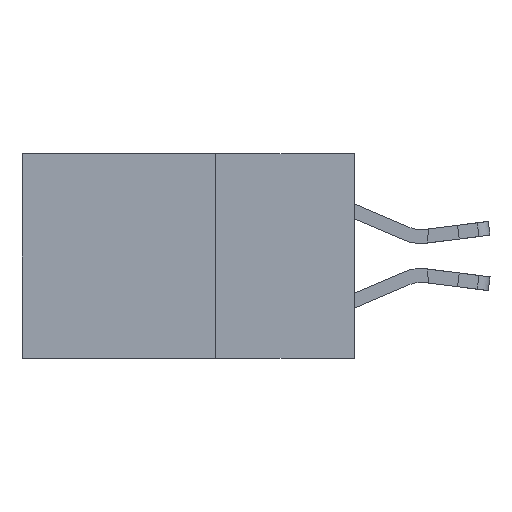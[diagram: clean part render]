
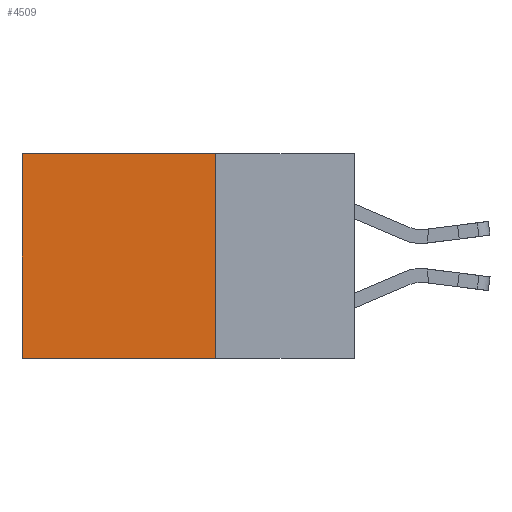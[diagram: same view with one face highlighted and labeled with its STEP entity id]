
A CAD part, left-side view. The second image highlights one B-rep face of the part: STEP entity #4509.
In plain terms, the highlighted planar face has unit normal (-1, 0, 0).
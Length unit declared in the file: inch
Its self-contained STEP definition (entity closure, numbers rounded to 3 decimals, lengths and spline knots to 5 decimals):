
#1687 = VERTEX_POINT ( 'NONE', #14600 ) ;
#2316 = EDGE_CURVE ( 'NONE', #16230, #3659, #2641, .T. ) ;
#2641 = LINE ( 'NONE', #6997, #9275 ) ;
#3416 = LINE ( 'NONE', #8461, #14261 ) ;
#3659 = VERTEX_POINT ( 'NONE', #3979 ) ;
#3664 = ORIENTED_EDGE ( 'NONE', *, *, #3799, .F. ) ;
#3799 = EDGE_CURVE ( 'NONE', #1687, #16230, #14791, .T. ) ;
#3826 = LINE ( 'NONE', #16804, #14677 ) ;
#3979 = CARTESIAN_POINT ( 'NONE',  ( 0.2615, 0.6, -0.37 ) ) ;
#4509 = ADVANCED_FACE ( 'NONE', ( #9915 ), #16626, .F. ) ;
#4846 = ORIENTED_EDGE ( 'NONE', *, *, #7621, .T. ) ;
#5616 = ORIENTED_EDGE ( 'NONE', *, *, #6507, .T. ) ;
#6488 = CARTESIAN_POINT ( 'NONE',  ( 0.2615, 0.25, -0.37 ) ) ;
#6507 = EDGE_CURVE ( 'NONE', #15084, #3659, #3416, .T. ) ;
#6636 = CARTESIAN_POINT ( 'NONE',  ( 0.2615, 0.25, -0.37 ) ) ;
#6684 = DIRECTION ( 'NONE',  ( 0., 1., 0. ) ) ;
#6997 = CARTESIAN_POINT ( 'NONE',  ( 0.2615, 0.25, -0.37 ) ) ;
#7621 = EDGE_CURVE ( 'NONE', #1687, #15084, #3826, .T. ) ;
#7877 = DIRECTION ( 'NONE',  ( 0., 0., -1. ) ) ;
#8461 = CARTESIAN_POINT ( 'NONE',  ( 0.2615, 0.6, -0.37 ) ) ;
#9275 = VECTOR ( 'NONE', #6684, 39.37008 ) ;
#9915 = FACE_OUTER_BOUND ( 'NONE', #13789, .T. ) ;
#10593 = AXIS2_PLACEMENT_3D ( 'NONE', #6488, #16431, #12468 ) ;
#11873 = DIRECTION ( 'NONE',  ( 0., 0., -1. ) ) ;
#12341 = ORIENTED_EDGE ( 'NONE', *, *, #2316, .F. ) ;
#12468 = DIRECTION ( 'NONE',  ( 0., 0., -1. ) ) ;
#12667 = CARTESIAN_POINT ( 'NONE',  ( 0.2615, 0.25, -0.37 ) ) ;
#13789 = EDGE_LOOP ( 'NONE', ( #5616, #12341, #3664, #4846 ) ) ;
#13917 = VECTOR ( 'NONE', #11873, 39.37008 ) ;
#14261 = VECTOR ( 'NONE', #7877, 39.37008 ) ;
#14600 = CARTESIAN_POINT ( 'NONE',  ( 0.2615, 0.25, 0. ) ) ;
#14677 = VECTOR ( 'NONE', #16785, 39.37008 ) ;
#14791 = LINE ( 'NONE', #6636, #13917 ) ;
#14942 = CARTESIAN_POINT ( 'NONE',  ( 0.2615, 0.6, 0. ) ) ;
#15084 = VERTEX_POINT ( 'NONE', #14942 ) ;
#16230 = VERTEX_POINT ( 'NONE', #12667 ) ;
#16431 = DIRECTION ( 'NONE',  ( 1., 0., 0. ) ) ;
#16626 = PLANE ( 'NONE',  #10593 ) ;
#16785 = DIRECTION ( 'NONE',  ( 0., 1., 0. ) ) ;
#16804 = CARTESIAN_POINT ( 'NONE',  ( 0.2615, 0.25, 0. ) ) ;
